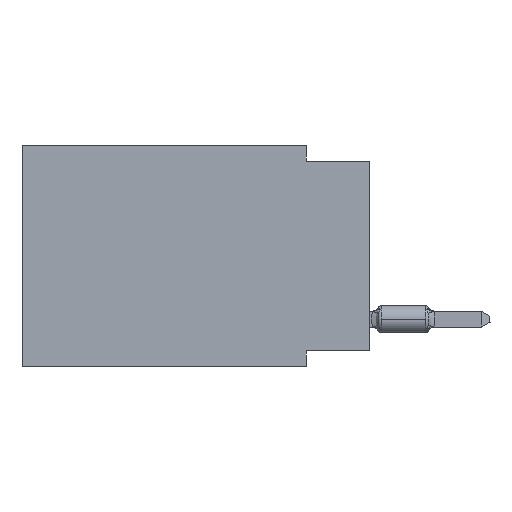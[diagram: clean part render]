
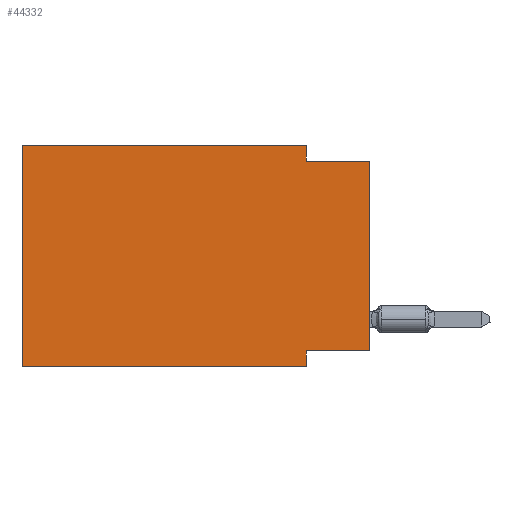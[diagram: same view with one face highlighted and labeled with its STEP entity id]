
A CAD part, left-side view. The second image highlights one B-rep face of the part: STEP entity #44332.
In plain terms, the highlighted planar face has unit normal (-1, 0, 0).
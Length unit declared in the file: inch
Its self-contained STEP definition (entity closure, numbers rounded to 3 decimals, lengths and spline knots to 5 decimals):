
#473 = DIRECTION ( 'NONE',  ( 0., 0., -1. ) ) ;
#1173 = ORIENTED_EDGE ( 'NONE', *, *, #60988, .T. ) ;
#1987 = LINE ( 'NONE', #20747, #17902 ) ;
#2291 = DIRECTION ( 'NONE',  ( 0., -1., 0. ) ) ;
#2488 = DIRECTION ( 'NONE',  ( 0., 0., -1. ) ) ;
#3408 = LINE ( 'NONE', #40605, #17601 ) ;
#6712 = VERTEX_POINT ( 'NONE', #39786 ) ;
#6734 = EDGE_CURVE ( 'NONE', #27612, #6712, #34164, .T. ) ;
#8869 = CARTESIAN_POINT ( 'NONE',  ( 0., 0.55, 0. ) ) ;
#9168 = VERTEX_POINT ( 'NONE', #13797 ) ;
#9294 = CARTESIAN_POINT ( 'NONE',  ( 0., 0., 0. ) ) ;
#9607 = DIRECTION ( 'NONE',  ( 0., 0., 1. ) ) ;
#10077 = EDGE_CURVE ( 'NONE', #15212, #27612, #32078, .T. ) ;
#10261 = DIRECTION ( 'NONE',  ( 0., 1., 0. ) ) ;
#11428 = ORIENTED_EDGE ( 'NONE', *, *, #52148, .F. ) ;
#13797 = CARTESIAN_POINT ( 'NONE',  ( 0., 0.55, 0. ) ) ;
#14661 = VECTOR ( 'NONE', #10261, 39.37008 ) ;
#15212 = VERTEX_POINT ( 'NONE', #19672 ) ;
#15773 = FACE_OUTER_BOUND ( 'NONE', #42541, .T. ) ;
#16257 = CARTESIAN_POINT ( 'NONE',  ( 0., 0.55, -0.35 ) ) ;
#17601 = VECTOR ( 'NONE', #2488, 39.37008 ) ;
#17902 = VECTOR ( 'NONE', #2291, 39.37008 ) ;
#18248 = LINE ( 'NONE', #8869, #41692 ) ;
#19672 = CARTESIAN_POINT ( 'NONE',  ( 0., 0.1, 0. ) ) ;
#20168 = VERTEX_POINT ( 'NONE', #34662 ) ;
#20747 = CARTESIAN_POINT ( 'NONE',  ( 0., 0.55, 0. ) ) ;
#24490 = VERTEX_POINT ( 'NONE', #50792 ) ;
#24502 = DIRECTION ( 'NONE',  ( 0., -1., 0. ) ) ;
#25689 = EDGE_CURVE ( 'NONE', #20168, #24490, #3408, .T. ) ;
#27504 = EDGE_CURVE ( 'NONE', #40205, #24490, #38010, .T. ) ;
#27612 = VERTEX_POINT ( 'NONE', #53584 ) ;
#27816 = CARTESIAN_POINT ( 'NONE',  ( 0., 0., -0.325 ) ) ;
#29521 = CARTESIAN_POINT ( 'NONE',  ( 0., 0.55, 0. ) ) ;
#32078 = LINE ( 'NONE', #50825, #57402 ) ;
#32445 = ORIENTED_EDGE ( 'NONE', *, *, #6734, .F. ) ;
#33306 = CARTESIAN_POINT ( 'NONE',  ( 0., 0.55, -0.35 ) ) ;
#33653 = ORIENTED_EDGE ( 'NONE', *, *, #27504, .T. ) ;
#34164 = LINE ( 'NONE', #53203, #57849 ) ;
#34662 = CARTESIAN_POINT ( 'NONE',  ( 0., 0.1, -0.325 ) ) ;
#37493 = VERTEX_POINT ( 'NONE', #27816 ) ;
#38010 = LINE ( 'NONE', #33306, #41713 ) ;
#38584 = PLANE ( 'NONE',  #54601 ) ;
#39786 = CARTESIAN_POINT ( 'NONE',  ( 0., 0., -0.025 ) ) ;
#39983 = EDGE_CURVE ( 'NONE', #40205, #9168, #18248, .T. ) ;
#40205 = VERTEX_POINT ( 'NONE', #16257 ) ;
#40605 = CARTESIAN_POINT ( 'NONE',  ( 0., 0.1, -0.35 ) ) ;
#40948 = ORIENTED_EDGE ( 'NONE', *, *, #10077, .F. ) ;
#41692 = VECTOR ( 'NONE', #51640, 39.37008 ) ;
#41713 = VECTOR ( 'NONE', #43008, 39.37008 ) ;
#42541 = EDGE_LOOP ( 'NONE', ( #1173, #32445, #40948, #11428, #46081, #33653, #44711, #45575 ) ) ;
#43008 = DIRECTION ( 'NONE',  ( 0., -1., 0. ) ) ;
#43331 = LINE ( 'NONE', #9294, #53261 ) ;
#43995 = LINE ( 'NONE', #49267, #14661 ) ;
#44332 = ADVANCED_FACE ( 'NONE', ( #15773 ), #38584, .F. ) ;
#44711 = ORIENTED_EDGE ( 'NONE', *, *, #25689, .F. ) ;
#45575 = ORIENTED_EDGE ( 'NONE', *, *, #49399, .F. ) ;
#46081 = ORIENTED_EDGE ( 'NONE', *, *, #39983, .F. ) ;
#46757 = DIRECTION ( 'NONE',  ( 0., 0., -1. ) ) ;
#49267 = CARTESIAN_POINT ( 'NONE',  ( 0., 0., -0.325 ) ) ;
#49399 = EDGE_CURVE ( 'NONE', #37493, #20168, #43995, .T. ) ;
#50792 = CARTESIAN_POINT ( 'NONE',  ( 0., 0.1, -0.35 ) ) ;
#50825 = CARTESIAN_POINT ( 'NONE',  ( 0., 0.1, 0. ) ) ;
#51640 = DIRECTION ( 'NONE',  ( 0., 0., 1. ) ) ;
#52148 = EDGE_CURVE ( 'NONE', #9168, #15212, #1987, .T. ) ;
#53203 = CARTESIAN_POINT ( 'NONE',  ( 0., 0., -0.025 ) ) ;
#53261 = VECTOR ( 'NONE', #9607, 39.37008 ) ;
#53542 = DIRECTION ( 'NONE',  ( 1., 0., 0. ) ) ;
#53584 = CARTESIAN_POINT ( 'NONE',  ( 0., 0.1, -0.025 ) ) ;
#54601 = AXIS2_PLACEMENT_3D ( 'NONE', #29521, #53542, #473 ) ;
#57402 = VECTOR ( 'NONE', #46757, 39.37008 ) ;
#57849 = VECTOR ( 'NONE', #24502, 39.37008 ) ;
#60988 = EDGE_CURVE ( 'NONE', #37493, #6712, #43331, .T. ) ;
